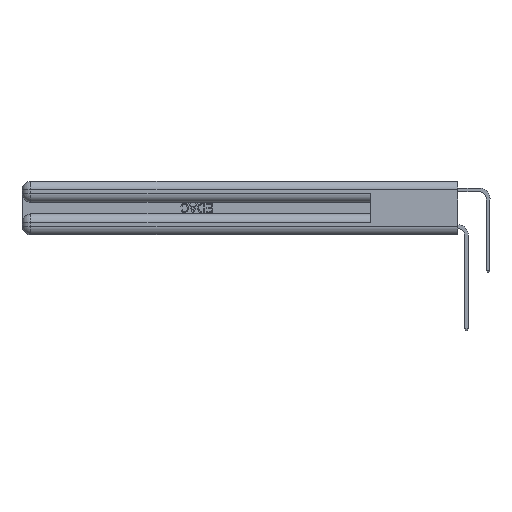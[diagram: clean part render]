
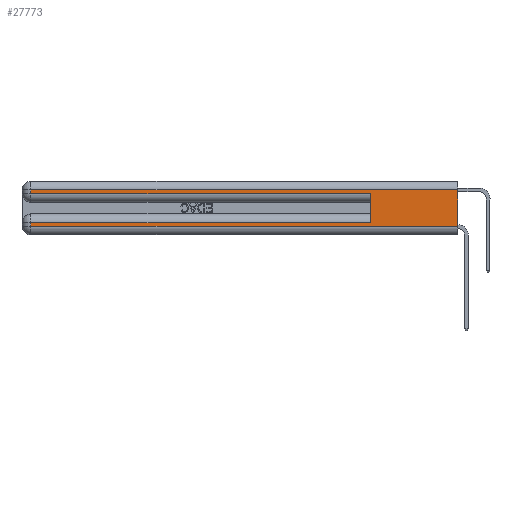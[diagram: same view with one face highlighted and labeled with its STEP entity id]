
A CAD part, left-side view. The second image highlights one B-rep face of the part: STEP entity #27773.
In plain terms, the highlighted planar face has unit normal (-1, 0, 0).
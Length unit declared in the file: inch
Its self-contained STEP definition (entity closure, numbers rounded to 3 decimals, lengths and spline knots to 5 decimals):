
#292 = VECTOR ( 'NONE', #19534, 39.37008 ) ;
#342 = VECTOR ( 'NONE', #15811, 39.37008 ) ;
#499 = CARTESIAN_POINT ( 'NONE',  ( 0., 0., 0.085 ) ) ;
#542 = LINE ( 'NONE', #7438, #4498 ) ;
#588 = ORIENTED_EDGE ( 'NONE', *, *, #15941, .T. ) ;
#730 = CARTESIAN_POINT ( 'NONE',  ( 0., 0., 0.31 ) ) ;
#1478 = CARTESIAN_POINT ( 'NONE',  ( 0., 0., 0.285 ) ) ;
#1556 = DIRECTION ( 'NONE',  ( 0., 0., -1. ) ) ;
#1676 = DIRECTION ( 'NONE',  ( 0., 0., -1. ) ) ;
#2018 = CARTESIAN_POINT ( 'NONE',  ( 0., 2.94, 0.37 ) ) ;
#2437 = FACE_OUTER_BOUND ( 'NONE', #7262, .T. ) ;
#3123 = ORIENTED_EDGE ( 'NONE', *, *, #23319, .T. ) ;
#3695 = ORIENTED_EDGE ( 'NONE', *, *, #16544, .T. ) ;
#3984 = CARTESIAN_POINT ( 'NONE',  ( 0., 0.6, 0.145 ) ) ;
#4498 = VECTOR ( 'NONE', #1676, 39.37008 ) ;
#4797 = CARTESIAN_POINT ( 'NONE',  ( 0., 0., 0.06 ) ) ;
#5153 = VERTEX_POINT ( 'NONE', #18888 ) ;
#5483 = VERTEX_POINT ( 'NONE', #10454 ) ;
#6221 = CARTESIAN_POINT ( 'NONE',  ( 0., 2.94, 0.37 ) ) ;
#6563 = LINE ( 'NONE', #29331, #11238 ) ;
#7262 = EDGE_LOOP ( 'NONE', ( #9579, #3695, #14289, #588, #10395, #26275, #16380, #3123 ) ) ;
#7296 = VECTOR ( 'NONE', #1556, 39.37008 ) ;
#7438 = CARTESIAN_POINT ( 'NONE',  ( 0., 0., 0.37 ) ) ;
#7873 = CARTESIAN_POINT ( 'NONE',  ( 0., 2.94, 0.285 ) ) ;
#8139 = AXIS2_PLACEMENT_3D ( 'NONE', #9944, #17053, #12446 ) ;
#9254 = CARTESIAN_POINT ( 'NONE',  ( 0., 2.94, 0.31 ) ) ;
#9439 = EDGE_CURVE ( 'NONE', #28059, #17012, #542, .T. ) ;
#9579 = ORIENTED_EDGE ( 'NONE', *, *, #9439, .F. ) ;
#9803 = CARTESIAN_POINT ( 'NONE',  ( 0., 2.94, 0.06 ) ) ;
#9944 = CARTESIAN_POINT ( 'NONE',  ( 0., 0., 0.37 ) ) ;
#10395 = ORIENTED_EDGE ( 'NONE', *, *, #12611, .F. ) ;
#10454 = CARTESIAN_POINT ( 'NONE',  ( 0., 2.94, 0.085 ) ) ;
#11238 = VECTOR ( 'NONE', #14422, 39.37008 ) ;
#11689 = LINE ( 'NONE', #2018, #292 ) ;
#11976 = LINE ( 'NONE', #6221, #7296 ) ;
#12018 = PLANE ( 'NONE',  #8139 ) ;
#12102 = VERTEX_POINT ( 'NONE', #9803 ) ;
#12446 = DIRECTION ( 'NONE',  ( 0., 0., -1. ) ) ;
#12611 = EDGE_CURVE ( 'NONE', #13715, #5153, #27345, .T. ) ;
#12845 = VERTEX_POINT ( 'NONE', #7873 ) ;
#13700 = EDGE_CURVE ( 'NONE', #13715, #5483, #14868, .T. ) ;
#13715 = VERTEX_POINT ( 'NONE', #18781 ) ;
#13890 = DIRECTION ( 'NONE',  ( 0., 1., 0. ) ) ;
#14289 = ORIENTED_EDGE ( 'NONE', *, *, #21063, .T. ) ;
#14422 = DIRECTION ( 'NONE',  ( 0., -1., 0. ) ) ;
#14868 = LINE ( 'NONE', #499, #16791 ) ;
#15811 = DIRECTION ( 'NONE',  ( 0., 1., 0. ) ) ;
#15941 = EDGE_CURVE ( 'NONE', #12845, #5153, #27363, .T. ) ;
#16380 = ORIENTED_EDGE ( 'NONE', *, *, #23724, .T. ) ;
#16445 = LINE ( 'NONE', #730, #342 ) ;
#16544 = EDGE_CURVE ( 'NONE', #28059, #26117, #16445, .T. ) ;
#16791 = VECTOR ( 'NONE', #13890, 39.37008 ) ;
#17012 = VERTEX_POINT ( 'NONE', #4797 ) ;
#17053 = DIRECTION ( 'NONE',  ( 1., 0., 0. ) ) ;
#18781 = CARTESIAN_POINT ( 'NONE',  ( 0., 0.6, 0.085 ) ) ;
#18888 = CARTESIAN_POINT ( 'NONE',  ( 0., 0.6, 0.285 ) ) ;
#19534 = DIRECTION ( 'NONE',  ( 0., 0., -1. ) ) ;
#20758 = VECTOR ( 'NONE', #21131, 39.37008 ) ;
#21063 = EDGE_CURVE ( 'NONE', #26117, #12845, #11689, .T. ) ;
#21131 = DIRECTION ( 'NONE',  ( 0., 0., 1. ) ) ;
#23319 = EDGE_CURVE ( 'NONE', #12102, #17012, #6563, .T. ) ;
#23724 = EDGE_CURVE ( 'NONE', #5483, #12102, #11976, .T. ) ;
#25177 = DIRECTION ( 'NONE',  ( 0., -1., 0. ) ) ;
#26073 = CARTESIAN_POINT ( 'NONE',  ( 0., 0., 0.31 ) ) ;
#26117 = VERTEX_POINT ( 'NONE', #9254 ) ;
#26275 = ORIENTED_EDGE ( 'NONE', *, *, #13700, .T. ) ;
#27345 = LINE ( 'NONE', #3984, #20758 ) ;
#27363 = LINE ( 'NONE', #1478, #28554 ) ;
#27773 = ADVANCED_FACE ( 'NONE', ( #2437 ), #12018, .F. ) ;
#28059 = VERTEX_POINT ( 'NONE', #26073 ) ;
#28554 = VECTOR ( 'NONE', #25177, 39.37008 ) ;
#29331 = CARTESIAN_POINT ( 'NONE',  ( 0., 0., 0.06 ) ) ;
